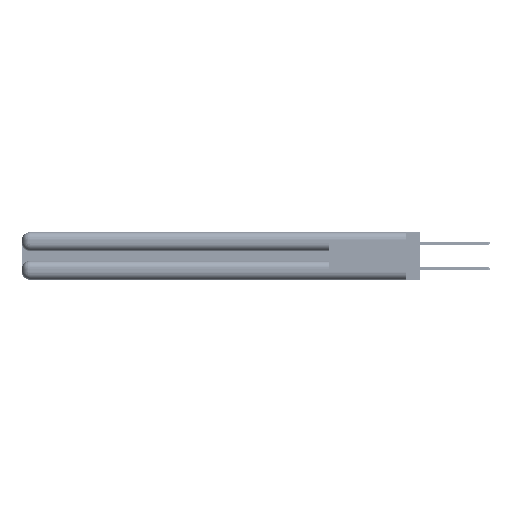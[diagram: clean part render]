
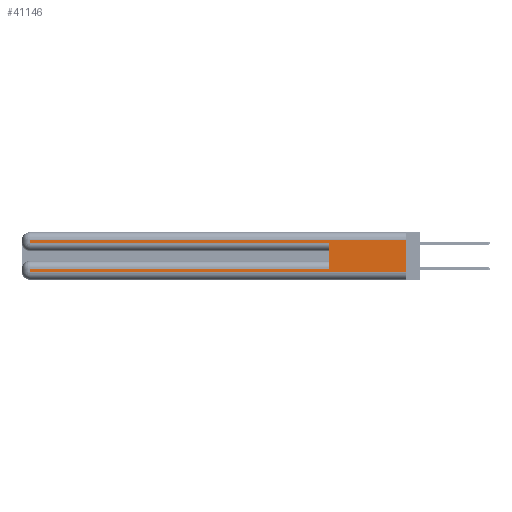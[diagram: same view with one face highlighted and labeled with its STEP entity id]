
A CAD part, left-side view. The second image highlights one B-rep face of the part: STEP entity #41146.
In plain terms, the highlighted planar face has unit normal (-1, 0, 0).
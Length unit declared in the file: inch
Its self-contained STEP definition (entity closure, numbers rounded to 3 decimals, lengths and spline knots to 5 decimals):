
#145 = DIRECTION ( 'NONE',  ( 0., -1., 0. ) ) ;
#493 = VECTOR ( 'NONE', #35048, 39.37008 ) ;
#1768 = ORIENTED_EDGE ( 'NONE', *, *, #48302, .F. ) ;
#1777 = LINE ( 'NONE', #26786, #493 ) ;
#2373 = ORIENTED_EDGE ( 'NONE', *, *, #36725, .F. ) ;
#2950 = EDGE_CURVE ( 'NONE', #12368, #38668, #13630, .T. ) ;
#3885 = VECTOR ( 'NONE', #145, 39.37008 ) ;
#4874 = LINE ( 'NONE', #33085, #36547 ) ;
#5354 = CARTESIAN_POINT ( 'NONE',  ( 0., 0., 0.31 ) ) ;
#6165 = PLANE ( 'NONE',  #11748 ) ;
#6359 = DIRECTION ( 'NONE',  ( 1., 0., 0. ) ) ;
#8158 = CARTESIAN_POINT ( 'NONE',  ( 0., 0., 0.06 ) ) ;
#8324 = DIRECTION ( 'NONE',  ( 0., 0., -1. ) ) ;
#8386 = VECTOR ( 'NONE', #49541, 39.37008 ) ;
#11748 = AXIS2_PLACEMENT_3D ( 'NONE', #31127, #6359, #35261 ) ;
#11784 = VERTEX_POINT ( 'NONE', #35379 ) ;
#12368 = VERTEX_POINT ( 'NONE', #35145 ) ;
#13630 = LINE ( 'NONE', #41420, #3885 ) ;
#14246 = VERTEX_POINT ( 'NONE', #5354 ) ;
#14808 = LINE ( 'NONE', #48462, #46333 ) ;
#14901 = LINE ( 'NONE', #50892, #23328 ) ;
#14915 = CARTESIAN_POINT ( 'NONE',  ( 0., 0.6, 0.285 ) ) ;
#17449 = EDGE_CURVE ( 'NONE', #25715, #45107, #19460, .T. ) ;
#18631 = ORIENTED_EDGE ( 'NONE', *, *, #41300, .T. ) ;
#18826 = CARTESIAN_POINT ( 'NONE',  ( 0., 2.94, 0.085 ) ) ;
#19460 = LINE ( 'NONE', #8158, #8386 ) ;
#19771 = CARTESIAN_POINT ( 'NONE',  ( 0., 2.94, 0.31 ) ) ;
#21257 = EDGE_CURVE ( 'NONE', #27654, #25715, #1777, .T. ) ;
#22619 = FACE_OUTER_BOUND ( 'NONE', #37574, .T. ) ;
#23328 = VECTOR ( 'NONE', #30489, 39.37008 ) ;
#25308 = CARTESIAN_POINT ( 'NONE',  ( 0., 0., 0.31 ) ) ;
#25715 = VERTEX_POINT ( 'NONE', #49881 ) ;
#26786 = CARTESIAN_POINT ( 'NONE',  ( 0., 2.94, 0.37 ) ) ;
#27654 = VERTEX_POINT ( 'NONE', #18826 ) ;
#27685 = ORIENTED_EDGE ( 'NONE', *, *, #39467, .T. ) ;
#28958 = ORIENTED_EDGE ( 'NONE', *, *, #21257, .T. ) ;
#29555 = CARTESIAN_POINT ( 'NONE',  ( 0., 0., 0.06 ) ) ;
#30489 = DIRECTION ( 'NONE',  ( 0., 0., 1. ) ) ;
#31127 = CARTESIAN_POINT ( 'NONE',  ( 0., 0., 0.37 ) ) ;
#33085 = CARTESIAN_POINT ( 'NONE',  ( 0., 0., 0.37 ) ) ;
#33447 = ORIENTED_EDGE ( 'NONE', *, *, #2950, .T. ) ;
#33678 = VECTOR ( 'NONE', #36639, 39.37008 ) ;
#35048 = DIRECTION ( 'NONE',  ( 0., 0., -1. ) ) ;
#35145 = CARTESIAN_POINT ( 'NONE',  ( 0., 2.94, 0.285 ) ) ;
#35261 = DIRECTION ( 'NONE',  ( 0., 0., -1. ) ) ;
#35379 = CARTESIAN_POINT ( 'NONE',  ( 0., 0.6, 0.085 ) ) ;
#35503 = EDGE_CURVE ( 'NONE', #14246, #51932, #41140, .T. ) ;
#36547 = VECTOR ( 'NONE', #8324, 39.37008 ) ;
#36639 = DIRECTION ( 'NONE',  ( 0., 1., 0. ) ) ;
#36725 = EDGE_CURVE ( 'NONE', #14246, #45107, #4874, .T. ) ;
#37574 = EDGE_LOOP ( 'NONE', ( #2373, #39201, #18631, #33447, #1768, #27685, #28958, #50730 ) ) ;
#38668 = VERTEX_POINT ( 'NONE', #14915 ) ;
#39201 = ORIENTED_EDGE ( 'NONE', *, *, #35503, .T. ) ;
#39467 = EDGE_CURVE ( 'NONE', #11784, #27654, #44551, .T. ) ;
#39873 = VECTOR ( 'NONE', #41585, 39.37008 ) ;
#41140 = LINE ( 'NONE', #25308, #39873 ) ;
#41146 = ADVANCED_FACE ( 'NONE', ( #22619 ), #6165, .F. ) ;
#41300 = EDGE_CURVE ( 'NONE', #51932, #12368, #14808, .T. ) ;
#41420 = CARTESIAN_POINT ( 'NONE',  ( 0., 0., 0.285 ) ) ;
#41585 = DIRECTION ( 'NONE',  ( 0., 1., 0. ) ) ;
#44551 = LINE ( 'NONE', #44676, #33678 ) ;
#44676 = CARTESIAN_POINT ( 'NONE',  ( 0., 0., 0.085 ) ) ;
#45107 = VERTEX_POINT ( 'NONE', #29555 ) ;
#46333 = VECTOR ( 'NONE', #48290, 39.37008 ) ;
#48290 = DIRECTION ( 'NONE',  ( 0., 0., -1. ) ) ;
#48302 = EDGE_CURVE ( 'NONE', #11784, #38668, #14901, .T. ) ;
#48462 = CARTESIAN_POINT ( 'NONE',  ( 0., 2.94, 0.37 ) ) ;
#49541 = DIRECTION ( 'NONE',  ( 0., -1., 0. ) ) ;
#49881 = CARTESIAN_POINT ( 'NONE',  ( 0., 2.94, 0.06 ) ) ;
#50730 = ORIENTED_EDGE ( 'NONE', *, *, #17449, .T. ) ;
#50892 = CARTESIAN_POINT ( 'NONE',  ( 0., 0.6, 0.145 ) ) ;
#51932 = VERTEX_POINT ( 'NONE', #19771 ) ;
